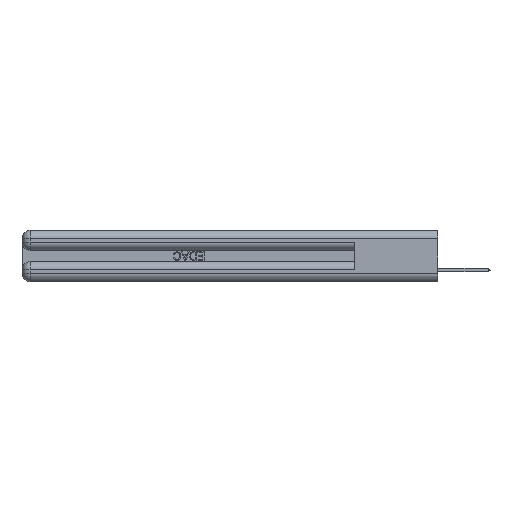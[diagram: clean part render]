
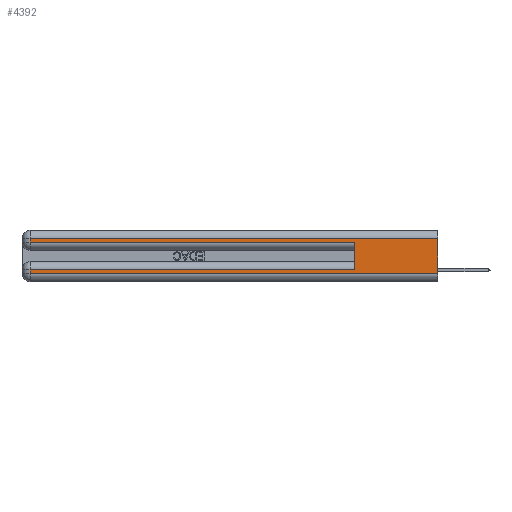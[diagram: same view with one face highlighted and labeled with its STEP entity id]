
A CAD part, left-side view. The second image highlights one B-rep face of the part: STEP entity #4392.
In plain terms, the highlighted planar face has unit normal (-1, 0, 0).
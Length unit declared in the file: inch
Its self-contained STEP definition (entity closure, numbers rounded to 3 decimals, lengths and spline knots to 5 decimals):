
#489 = EDGE_CURVE ( 'NONE', #28943, #4520, #17694, .T. ) ;
#1383 = ORIENTED_EDGE ( 'NONE', *, *, #27279, .T. ) ;
#1916 = VECTOR ( 'NONE', #6003, 39.37008 ) ;
#1978 = EDGE_CURVE ( 'NONE', #24557, #23379, #17534, .T. ) ;
#3858 = ORIENTED_EDGE ( 'NONE', *, *, #10101, .T. ) ;
#4392 = ADVANCED_FACE ( 'NONE', ( #6002 ), #12378, .F. ) ;
#4520 = VERTEX_POINT ( 'NONE', #11844 ) ;
#4535 = DIRECTION ( 'NONE',  ( 0., 1., 0. ) ) ;
#5551 = CARTESIAN_POINT ( 'NONE',  ( 0., 0.6, 0.285 ) ) ;
#5908 = LINE ( 'NONE', #20904, #25414 ) ;
#6002 = FACE_OUTER_BOUND ( 'NONE', #9336, .T. ) ;
#6003 = DIRECTION ( 'NONE',  ( 0., -1., 0. ) ) ;
#8491 = VERTEX_POINT ( 'NONE', #28197 ) ;
#9262 = CARTESIAN_POINT ( 'NONE',  ( 0., 0., 0.085 ) ) ;
#9336 = EDGE_LOOP ( 'NONE', ( #28166, #3858, #35761, #36713, #24737, #1383, #31842, #35676 ) ) ;
#9529 = LINE ( 'NONE', #33704, #18997 ) ;
#9775 = VECTOR ( 'NONE', #33625, 39.37008 ) ;
#9874 = CARTESIAN_POINT ( 'NONE',  ( 0., 2.94, 0.285 ) ) ;
#10101 = EDGE_CURVE ( 'NONE', #28943, #26303, #38098, .T. ) ;
#10418 = DIRECTION ( 'NONE',  ( 0., 0., 1. ) ) ;
#10763 = VECTOR ( 'NONE', #4535, 39.37008 ) ;
#11236 = EDGE_CURVE ( 'NONE', #26303, #24557, #5908, .T. ) ;
#11844 = CARTESIAN_POINT ( 'NONE',  ( 0., 0., 0.06 ) ) ;
#12378 = PLANE ( 'NONE',  #17667 ) ;
#13516 = CARTESIAN_POINT ( 'NONE',  ( 0., 2.94, 0.31 ) ) ;
#14485 = VECTOR ( 'NONE', #21861, 39.37008 ) ;
#15118 = LINE ( 'NONE', #26026, #1916 ) ;
#16099 = EDGE_CURVE ( 'NONE', #19178, #23379, #9529, .T. ) ;
#16763 = CARTESIAN_POINT ( 'NONE',  ( 0., 0.6, 0.085 ) ) ;
#16925 = LINE ( 'NONE', #9262, #42177 ) ;
#17534 = LINE ( 'NONE', #37134, #40668 ) ;
#17667 = AXIS2_PLACEMENT_3D ( 'NONE', #35907, #39280, #19134 ) ;
#17694 = LINE ( 'NONE', #42178, #14485 ) ;
#18387 = CARTESIAN_POINT ( 'NONE',  ( 0., 2.94, 0.06 ) ) ;
#18750 = VERTEX_POINT ( 'NONE', #18387 ) ;
#18856 = CARTESIAN_POINT ( 'NONE',  ( 0., 2.94, 0.37 ) ) ;
#18997 = VECTOR ( 'NONE', #10418, 39.37008 ) ;
#19134 = DIRECTION ( 'NONE',  ( 0., 0., -1. ) ) ;
#19178 = VERTEX_POINT ( 'NONE', #16763 ) ;
#20904 = CARTESIAN_POINT ( 'NONE',  ( 0., 2.94, 0.37 ) ) ;
#21861 = DIRECTION ( 'NONE',  ( 0., 0., -1. ) ) ;
#23379 = VERTEX_POINT ( 'NONE', #5551 ) ;
#24557 = VERTEX_POINT ( 'NONE', #9874 ) ;
#24737 = ORIENTED_EDGE ( 'NONE', *, *, #16099, .F. ) ;
#25414 = VECTOR ( 'NONE', #41346, 39.37008 ) ;
#26026 = CARTESIAN_POINT ( 'NONE',  ( 0., 0., 0.06 ) ) ;
#26303 = VERTEX_POINT ( 'NONE', #13516 ) ;
#26965 = CARTESIAN_POINT ( 'NONE',  ( 0., 0., 0.31 ) ) ;
#27153 = DIRECTION ( 'NONE',  ( 0., -1., 0. ) ) ;
#27279 = EDGE_CURVE ( 'NONE', #19178, #8491, #16925, .T. ) ;
#28166 = ORIENTED_EDGE ( 'NONE', *, *, #489, .F. ) ;
#28197 = CARTESIAN_POINT ( 'NONE',  ( 0., 2.94, 0.085 ) ) ;
#28943 = VERTEX_POINT ( 'NONE', #35272 ) ;
#29327 = DIRECTION ( 'NONE',  ( 0., 1., 0. ) ) ;
#31842 = ORIENTED_EDGE ( 'NONE', *, *, #40764, .T. ) ;
#33625 = DIRECTION ( 'NONE',  ( 0., 0., -1. ) ) ;
#33704 = CARTESIAN_POINT ( 'NONE',  ( 0., 0.6, 0.145 ) ) ;
#35272 = CARTESIAN_POINT ( 'NONE',  ( 0., 0., 0.31 ) ) ;
#35676 = ORIENTED_EDGE ( 'NONE', *, *, #40304, .T. ) ;
#35761 = ORIENTED_EDGE ( 'NONE', *, *, #11236, .T. ) ;
#35907 = CARTESIAN_POINT ( 'NONE',  ( 0., 0., 0.37 ) ) ;
#36713 = ORIENTED_EDGE ( 'NONE', *, *, #1978, .T. ) ;
#37134 = CARTESIAN_POINT ( 'NONE',  ( 0., 0., 0.285 ) ) ;
#38098 = LINE ( 'NONE', #26965, #10763 ) ;
#39280 = DIRECTION ( 'NONE',  ( 1., 0., 0. ) ) ;
#39782 = LINE ( 'NONE', #18856, #9775 ) ;
#40304 = EDGE_CURVE ( 'NONE', #18750, #4520, #15118, .T. ) ;
#40668 = VECTOR ( 'NONE', #27153, 39.37008 ) ;
#40764 = EDGE_CURVE ( 'NONE', #8491, #18750, #39782, .T. ) ;
#41346 = DIRECTION ( 'NONE',  ( 0., 0., -1. ) ) ;
#42177 = VECTOR ( 'NONE', #29327, 39.37008 ) ;
#42178 = CARTESIAN_POINT ( 'NONE',  ( 0., 0., 0.37 ) ) ;
